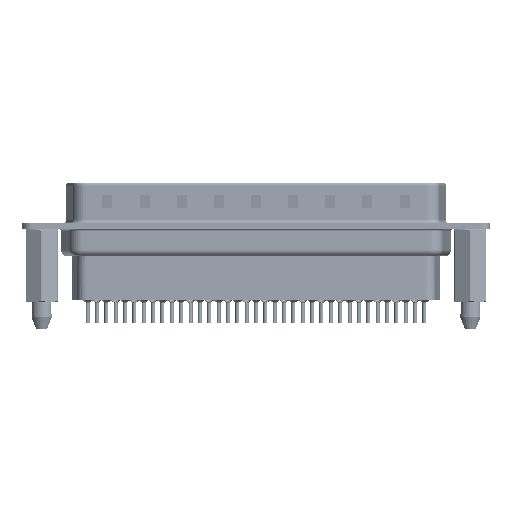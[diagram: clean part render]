
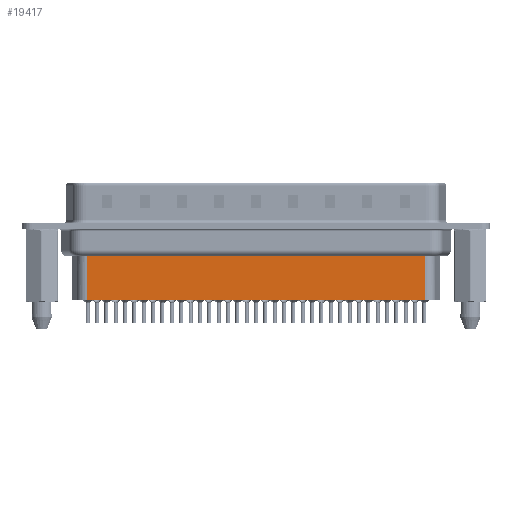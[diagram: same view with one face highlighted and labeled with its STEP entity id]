
A CAD part, front view. The second image highlights one B-rep face of the part: STEP entity #19417.
In plain terms, the highlighted planar face has unit normal (0, -1, 0).
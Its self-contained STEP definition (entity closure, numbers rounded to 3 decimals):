
#601 = DIRECTION ( 'NONE',  ( 0., -1., 0. ) ) ;
#1066 = CARTESIAN_POINT ( 'NONE',  ( 56.794, -3.5, -10.95 ) ) ;
#1550 = LINE ( 'NONE', #19513, #1876 ) ;
#1876 = VECTOR ( 'NONE', #32295, 1000. ) ;
#2780 = EDGE_CURVE ( 'NONE', #32189, #6763, #31254, .T. ) ;
#3402 = EDGE_LOOP ( 'NONE', ( #15210, #5223, #21249, #6474 ) ) ;
#4699 = CARTESIAN_POINT ( 'NONE',  ( 6.706, -3.5, -3.1 ) ) ;
#4934 = LINE ( 'NONE', #24906, #26094 ) ;
#5223 = ORIENTED_EDGE ( 'NONE', *, *, #18039, .T. ) ;
#5970 = PLANE ( 'NONE',  #29279 ) ;
#6474 = ORIENTED_EDGE ( 'NONE', *, *, #12540, .F. ) ;
#6763 = VERTEX_POINT ( 'NONE', #1066 ) ;
#8647 = DIRECTION ( 'NONE',  ( 1., 0., 0. ) ) ;
#11251 = VECTOR ( 'NONE', #14934, 1000. ) ;
#12130 = DIRECTION ( 'NONE',  ( -1., 0., 0. ) ) ;
#12540 = EDGE_CURVE ( 'NONE', #6763, #29722, #4934, .T. ) ;
#12812 = CARTESIAN_POINT ( 'NONE',  ( 6.706, -3.5, -10.95 ) ) ;
#12957 = CARTESIAN_POINT ( 'NONE',  ( 56.794, -3.5, -3.1 ) ) ;
#13525 = CARTESIAN_POINT ( 'NONE',  ( 6.706, -3.5, -3.1 ) ) ;
#14934 = DIRECTION ( 'NONE',  ( 0., 0., -1. ) ) ;
#15210 = ORIENTED_EDGE ( 'NONE', *, *, #2780, .F. ) ;
#16275 = VERTEX_POINT ( 'NONE', #27238 ) ;
#17120 = LINE ( 'NONE', #4699, #11251 ) ;
#18039 = EDGE_CURVE ( 'NONE', #32189, #16275, #1550, .T. ) ;
#18228 = FACE_OUTER_BOUND ( 'NONE', #3402, .T. ) ;
#19417 = ADVANCED_FACE ( 'NONE', ( #18228 ), #5970, .T. ) ;
#19513 = CARTESIAN_POINT ( 'NONE',  ( 6.459, -3.5, -4.097 ) ) ;
#19622 = VECTOR ( 'NONE', #23362, 1000. ) ;
#21249 = ORIENTED_EDGE ( 'NONE', *, *, #24391, .T. ) ;
#22536 = CARTESIAN_POINT ( 'NONE',  ( 56.794, -3.5, -4.097 ) ) ;
#23362 = DIRECTION ( 'NONE',  ( 0., 0., -1. ) ) ;
#24391 = EDGE_CURVE ( 'NONE', #16275, #29722, #17120, .T. ) ;
#24906 = CARTESIAN_POINT ( 'NONE',  ( 6.706, -3.5, -10.95 ) ) ;
#26094 = VECTOR ( 'NONE', #12130, 1000. ) ;
#27238 = CARTESIAN_POINT ( 'NONE',  ( 6.706, -3.5, -4.097 ) ) ;
#29279 = AXIS2_PLACEMENT_3D ( 'NONE', #13525, #601, #8647 ) ;
#29722 = VERTEX_POINT ( 'NONE', #12812 ) ;
#31254 = LINE ( 'NONE', #12957, #19622 ) ;
#32189 = VERTEX_POINT ( 'NONE', #22536 ) ;
#32295 = DIRECTION ( 'NONE',  ( -1., 0., 0. ) ) ;
